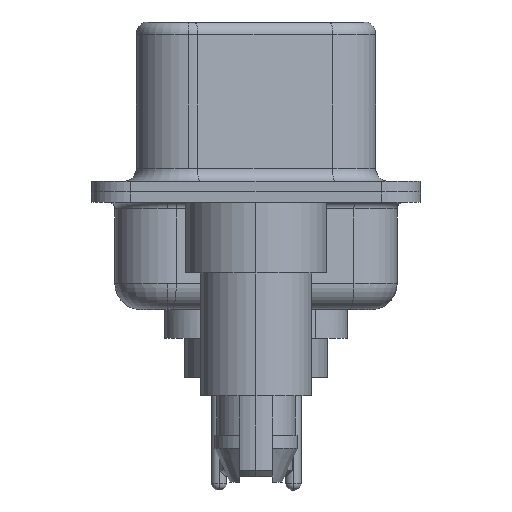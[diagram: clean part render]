
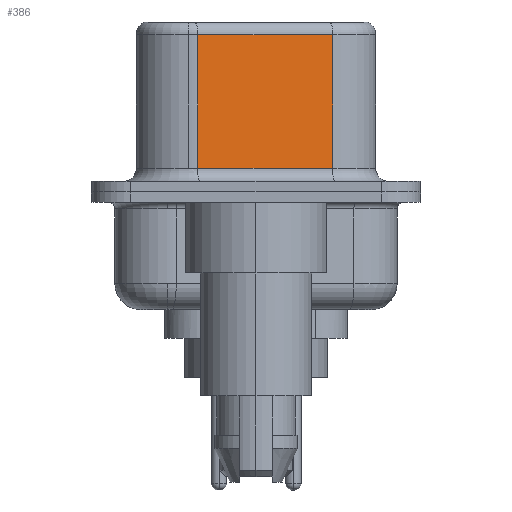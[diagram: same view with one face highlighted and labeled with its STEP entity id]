
A CAD part, left-side view. The second image highlights one B-rep face of the part: STEP entity #386.
In plain terms, the highlighted planar face has unit normal (-0.985, -0.174, 0).
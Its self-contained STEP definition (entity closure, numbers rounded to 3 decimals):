
#386 = ADVANCED_FACE ( 'NONE', ( #15126 ), #17062, .F. ) ;
#1313 = DIRECTION ( 'NONE',  ( 0., 0., -1. ) ) ;
#2139 = ORIENTED_EDGE ( 'NONE', *, *, #11711, .T. ) ;
#2561 = LINE ( 'NONE', #17768, #22721 ) ;
#5486 = DIRECTION ( 'NONE',  ( -0.174, 0.985, 0. ) ) ;
#5757 = CARTESIAN_POINT ( 'NONE',  ( 3.675, 2.233, 6.02 ) ) ;
#6406 = EDGE_CURVE ( 'NONE', #21535, #10305, #15358, .T. ) ;
#7448 = CARTESIAN_POINT ( 'NONE',  ( 4.585, -2.927, 6.52 ) ) ;
#7621 = DIRECTION ( 'NONE',  ( 0.985, 0.174, 0. ) ) ;
#7898 = AXIS2_PLACEMENT_3D ( 'NONE', #7448, #7621, #22948 ) ;
#8048 = EDGE_CURVE ( 'NONE', #16310, #10305, #2561, .T. ) ;
#8124 = DIRECTION ( 'NONE',  ( 0.174, -0.985, 0. ) ) ;
#9424 = VECTOR ( 'NONE', #17569, 1000. ) ;
#10019 = CARTESIAN_POINT ( 'NONE',  ( 3.675, 2.233, 0.9 ) ) ;
#10041 = CARTESIAN_POINT ( 'NONE',  ( 4.585, -2.927, 0.9 ) ) ;
#10305 = VERTEX_POINT ( 'NONE', #23818 ) ;
#11222 = VECTOR ( 'NONE', #8124, 1000. ) ;
#11711 = EDGE_CURVE ( 'NONE', #18458, #21535, #19461, .T. ) ;
#13459 = CARTESIAN_POINT ( 'NONE',  ( 4.585, -2.927, 6.02 ) ) ;
#13934 = LINE ( 'NONE', #22320, #16888 ) ;
#15126 = FACE_OUTER_BOUND ( 'NONE', #19100, .T. ) ;
#15358 = LINE ( 'NONE', #10041, #11222 ) ;
#15684 = CARTESIAN_POINT ( 'NONE',  ( 3.675, 2.233, 6.52 ) ) ;
#16310 = VERTEX_POINT ( 'NONE', #13459 ) ;
#16888 = VECTOR ( 'NONE', #5486, 1000. ) ;
#17062 = PLANE ( 'NONE',  #7898 ) ;
#17569 = DIRECTION ( 'NONE',  ( 0., 0., -1. ) ) ;
#17768 = CARTESIAN_POINT ( 'NONE',  ( 4.585, -2.927, 6.52 ) ) ;
#18239 = ORIENTED_EDGE ( 'NONE', *, *, #8048, .F. ) ;
#18458 = VERTEX_POINT ( 'NONE', #5757 ) ;
#18496 = ORIENTED_EDGE ( 'NONE', *, *, #23104, .T. ) ;
#19100 = EDGE_LOOP ( 'NONE', ( #18239, #18496, #2139, #20030 ) ) ;
#19461 = LINE ( 'NONE', #15684, #9424 ) ;
#20030 = ORIENTED_EDGE ( 'NONE', *, *, #6406, .T. ) ;
#21535 = VERTEX_POINT ( 'NONE', #10019 ) ;
#22320 = CARTESIAN_POINT ( 'NONE',  ( 4.585, -2.927, 6.02 ) ) ;
#22721 = VECTOR ( 'NONE', #1313, 1000. ) ;
#22948 = DIRECTION ( 'NONE',  ( -0.174, 0.985, 0. ) ) ;
#23104 = EDGE_CURVE ( 'NONE', #16310, #18458, #13934, .T. ) ;
#23818 = CARTESIAN_POINT ( 'NONE',  ( 4.585, -2.927, 0.9 ) ) ;
